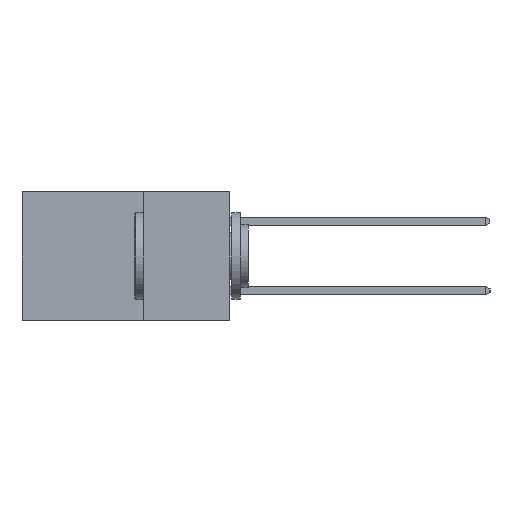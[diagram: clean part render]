
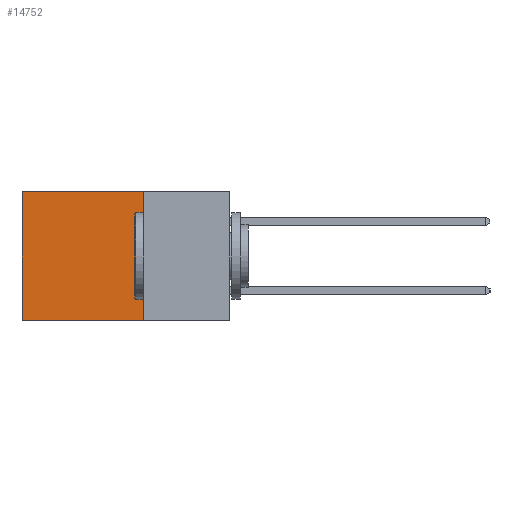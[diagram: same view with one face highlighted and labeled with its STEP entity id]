
A CAD part, left-side view. The second image highlights one B-rep face of the part: STEP entity #14752.
In plain terms, the highlighted planar face has unit normal (-1, 0, 0).
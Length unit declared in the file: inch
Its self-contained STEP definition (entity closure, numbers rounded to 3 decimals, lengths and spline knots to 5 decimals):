
#276 = ORIENTED_EDGE ( 'NONE', *, *, #11649, .T. ) ;
#712 = CARTESIAN_POINT ( 'NONE',  ( 0.2615, 0.25, -0.37 ) ) ;
#1703 = VECTOR ( 'NONE', #6901, 39.37008 ) ;
#1717 = VERTEX_POINT ( 'NONE', #10176 ) ;
#2290 = DIRECTION ( 'NONE',  ( 0., 0., -1. ) ) ;
#2648 = CARTESIAN_POINT ( 'NONE',  ( 0.2615, 0.25, -0.37 ) ) ;
#2969 = VERTEX_POINT ( 'NONE', #712 ) ;
#3386 = ORIENTED_EDGE ( 'NONE', *, *, #7349, .F. ) ;
#3444 = DIRECTION ( 'NONE',  ( 1., 0., 0. ) ) ;
#4342 = VECTOR ( 'NONE', #2290, 39.37008 ) ;
#4652 = PLANE ( 'NONE',  #11009 ) ;
#5457 = EDGE_LOOP ( 'NONE', ( #14852, #3386, #11741, #276 ) ) ;
#5949 = VECTOR ( 'NONE', #11232, 39.37008 ) ;
#6901 = DIRECTION ( 'NONE',  ( 0., 1., 0. ) ) ;
#7160 = VECTOR ( 'NONE', #7698, 39.37008 ) ;
#7349 = EDGE_CURVE ( 'NONE', #2969, #1717, #7554, .T. ) ;
#7554 = LINE ( 'NONE', #2648, #7160 ) ;
#7660 = CARTESIAN_POINT ( 'NONE',  ( 0.2615, 0.6, 0. ) ) ;
#7698 = DIRECTION ( 'NONE',  ( 0., 1., 0. ) ) ;
#8545 = CARTESIAN_POINT ( 'NONE',  ( 0.2615, 0.25, -0.37 ) ) ;
#9318 = LINE ( 'NONE', #14522, #5949 ) ;
#9734 = CARTESIAN_POINT ( 'NONE',  ( 0.2615, 0.25, -0.37 ) ) ;
#10176 = CARTESIAN_POINT ( 'NONE',  ( 0.2615, 0.6, -0.37 ) ) ;
#10590 = VERTEX_POINT ( 'NONE', #7660 ) ;
#11009 = AXIS2_PLACEMENT_3D ( 'NONE', #9734, #3444, #12175 ) ;
#11232 = DIRECTION ( 'NONE',  ( 0., 0., -1. ) ) ;
#11576 = FACE_OUTER_BOUND ( 'NONE', #5457, .T. ) ;
#11649 = EDGE_CURVE ( 'NONE', #13186, #10590, #14439, .T. ) ;
#11741 = ORIENTED_EDGE ( 'NONE', *, *, #13744, .F. ) ;
#12175 = DIRECTION ( 'NONE',  ( 0., 0., -1. ) ) ;
#12401 = CARTESIAN_POINT ( 'NONE',  ( 0.2615, 0.25, 0. ) ) ;
#13167 = EDGE_CURVE ( 'NONE', #10590, #1717, #9318, .T. ) ;
#13186 = VERTEX_POINT ( 'NONE', #12401 ) ;
#13744 = EDGE_CURVE ( 'NONE', #13186, #2969, #13802, .T. ) ;
#13802 = LINE ( 'NONE', #8545, #4342 ) ;
#14439 = LINE ( 'NONE', #15371, #1703 ) ;
#14522 = CARTESIAN_POINT ( 'NONE',  ( 0.2615, 0.6, -0.37 ) ) ;
#14752 = ADVANCED_FACE ( 'NONE', ( #11576 ), #4652, .F. ) ;
#14852 = ORIENTED_EDGE ( 'NONE', *, *, #13167, .T. ) ;
#15371 = CARTESIAN_POINT ( 'NONE',  ( 0.2615, 0.25, 0. ) ) ;
